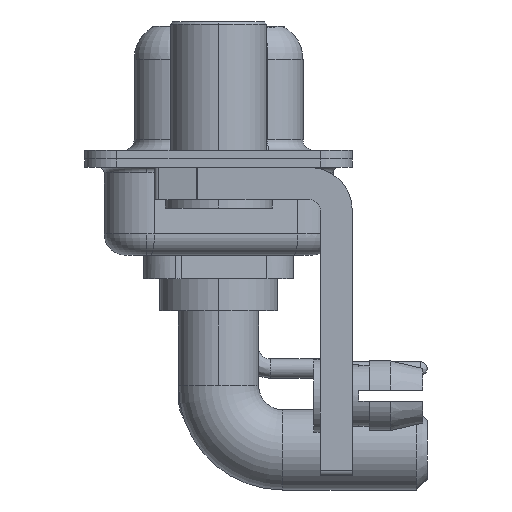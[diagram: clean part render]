
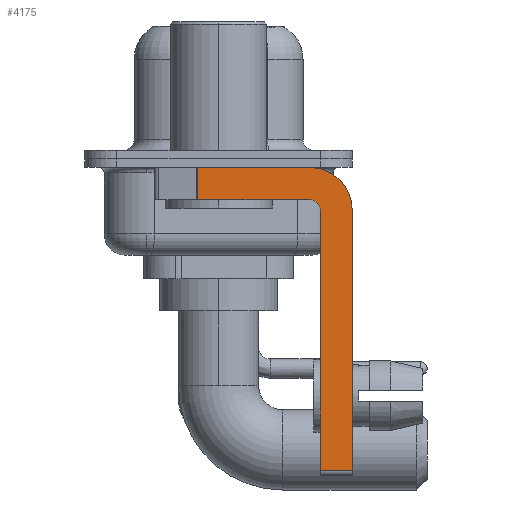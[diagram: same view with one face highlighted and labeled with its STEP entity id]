
A CAD part, left-side view. The second image highlights one B-rep face of the part: STEP entity #4175.
In plain terms, the highlighted planar face has unit normal (-1, 0, 0).
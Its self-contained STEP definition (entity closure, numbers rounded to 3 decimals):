
#1119 = ORIENTED_EDGE ( 'NONE', *, *, #23813, .T. ) ;
#1232 = CARTESIAN_POINT ( 'NONE',  ( -2.9, -4.25, -2.4 ) ) ;
#2039 = VERTEX_POINT ( 'NONE', #3082 ) ;
#2675 = CARTESIAN_POINT ( 'NONE',  ( -2.9, -4.75, -2.4 ) ) ;
#3079 = VERTEX_POINT ( 'NONE', #10028 ) ;
#3082 = CARTESIAN_POINT ( 'NONE',  ( -2.9, 0.978, -1.9 ) ) ;
#3207 = DIRECTION ( 'NONE',  ( 1., 0., 0. ) ) ;
#3347 = CARTESIAN_POINT ( 'NONE',  ( -2.9, -4.25, -1.9 ) ) ;
#4175 = ADVANCED_FACE ( 'NONE', ( #14173 ), #4944, .F. ) ;
#4270 = VERTEX_POINT ( 'NONE', #14654 ) ;
#4944 = PLANE ( 'NONE',  #5018 ) ;
#5018 = AXIS2_PLACEMENT_3D ( 'NONE', #1232, #3207, #8748 ) ;
#5119 = CARTESIAN_POINT ( 'NONE',  ( -2.9, 0.978, -0.4 ) ) ;
#5576 = DIRECTION ( 'NONE',  ( 0., 0., -1. ) ) ;
#5685 = VERTEX_POINT ( 'NONE', #18615 ) ;
#5725 = CARTESIAN_POINT ( 'NONE',  ( -2.9, -4.75, -14.8 ) ) ;
#6077 = LINE ( 'NONE', #5725, #24108 ) ;
#6092 = EDGE_LOOP ( 'NONE', ( #21932, #1119, #11904, #21109, #12220, #10313, #22774, #11377 ) ) ;
#6353 = AXIS2_PLACEMENT_3D ( 'NONE', #11463, #20855, #5576 ) ;
#7285 = LINE ( 'NONE', #3347, #11960 ) ;
#7549 = CIRCLE ( 'NONE', #6353, 2. ) ;
#7759 = EDGE_CURVE ( 'NONE', #4270, #19873, #7549, .T. ) ;
#7897 = LINE ( 'NONE', #22899, #8906 ) ;
#7976 = CIRCLE ( 'NONE', #8371, 0.5 ) ;
#8280 = DIRECTION ( 'NONE',  ( 0., 0., 1. ) ) ;
#8371 = AXIS2_PLACEMENT_3D ( 'NONE', #19504, #9771, #8280 ) ;
#8681 = CARTESIAN_POINT ( 'NONE',  ( -2.9, -6.25, -2.4 ) ) ;
#8747 = EDGE_CURVE ( 'NONE', #5685, #18491, #6077, .T. ) ;
#8748 = DIRECTION ( 'NONE',  ( 0., 0., -1. ) ) ;
#8906 = VECTOR ( 'NONE', #14274, 1000. ) ;
#9575 = CARTESIAN_POINT ( 'NONE',  ( -2.9, -6.25, -2.4 ) ) ;
#9771 = DIRECTION ( 'NONE',  ( -1., 0., 0. ) ) ;
#10028 = CARTESIAN_POINT ( 'NONE',  ( -2.9, -6.25, -14.55 ) ) ;
#10313 = ORIENTED_EDGE ( 'NONE', *, *, #11410, .T. ) ;
#11377 = ORIENTED_EDGE ( 'NONE', *, *, #7759, .F. ) ;
#11410 = EDGE_CURVE ( 'NONE', #5685, #3079, #19298, .T. ) ;
#11463 = CARTESIAN_POINT ( 'NONE',  ( -2.9, -4.25, -2.4 ) ) ;
#11638 = DIRECTION ( 'NONE',  ( 0., -1., 0. ) ) ;
#11762 = CARTESIAN_POINT ( 'NONE',  ( -2.9, -4.25, -14.55 ) ) ;
#11904 = ORIENTED_EDGE ( 'NONE', *, *, #22184, .F. ) ;
#11960 = VECTOR ( 'NONE', #22061, 1000. ) ;
#12084 = DIRECTION ( 'NONE',  ( 0., -1., 0. ) ) ;
#12220 = ORIENTED_EDGE ( 'NONE', *, *, #8747, .F. ) ;
#13565 = LINE ( 'NONE', #17517, #14395 ) ;
#14173 = FACE_OUTER_BOUND ( 'NONE', #6092, .T. ) ;
#14274 = DIRECTION ( 'NONE',  ( 0., 0., -1. ) ) ;
#14395 = VECTOR ( 'NONE', #12084, 1000. ) ;
#14654 = CARTESIAN_POINT ( 'NONE',  ( -2.9, -4.25, -0.4 ) ) ;
#15090 = EDGE_CURVE ( 'NONE', #16956, #4270, #13565, .T. ) ;
#15350 = CARTESIAN_POINT ( 'NONE',  ( -2.9, -4.25, -1.9 ) ) ;
#15452 = DIRECTION ( 'NONE',  ( 0., 0., 1. ) ) ;
#16321 = VECTOR ( 'NONE', #18954, 1000. ) ;
#16956 = VERTEX_POINT ( 'NONE', #5119 ) ;
#16971 = LINE ( 'NONE', #9575, #16321 ) ;
#17517 = CARTESIAN_POINT ( 'NONE',  ( -2.9, 3., -0.4 ) ) ;
#18491 = VERTEX_POINT ( 'NONE', #2675 ) ;
#18615 = CARTESIAN_POINT ( 'NONE',  ( -2.9, -4.75, -14.55 ) ) ;
#18954 = DIRECTION ( 'NONE',  ( 0., 0., -1. ) ) ;
#18964 = VERTEX_POINT ( 'NONE', #15350 ) ;
#19298 = LINE ( 'NONE', #11762, #20357 ) ;
#19357 = EDGE_CURVE ( 'NONE', #18491, #18964, #7976, .T. ) ;
#19504 = CARTESIAN_POINT ( 'NONE',  ( -2.9, -4.25, -2.4 ) ) ;
#19873 = VERTEX_POINT ( 'NONE', #8681 ) ;
#20357 = VECTOR ( 'NONE', #11638, 1000. ) ;
#20855 = DIRECTION ( 'NONE',  ( 1., 0., 0. ) ) ;
#21109 = ORIENTED_EDGE ( 'NONE', *, *, #19357, .F. ) ;
#21932 = ORIENTED_EDGE ( 'NONE', *, *, #15090, .F. ) ;
#22061 = DIRECTION ( 'NONE',  ( 0., 1., 0. ) ) ;
#22184 = EDGE_CURVE ( 'NONE', #18964, #2039, #7285, .T. ) ;
#22738 = EDGE_CURVE ( 'NONE', #19873, #3079, #16971, .T. ) ;
#22774 = ORIENTED_EDGE ( 'NONE', *, *, #22738, .F. ) ;
#22899 = CARTESIAN_POINT ( 'NONE',  ( -2.9, 0.978, -1.9 ) ) ;
#23813 = EDGE_CURVE ( 'NONE', #16956, #2039, #7897, .T. ) ;
#24108 = VECTOR ( 'NONE', #15452, 1000. ) ;
